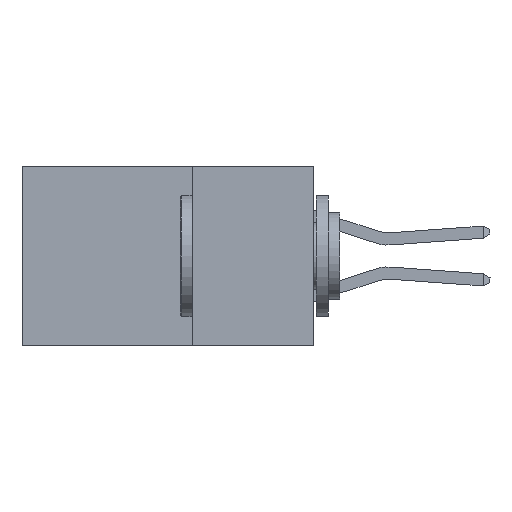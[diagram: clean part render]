
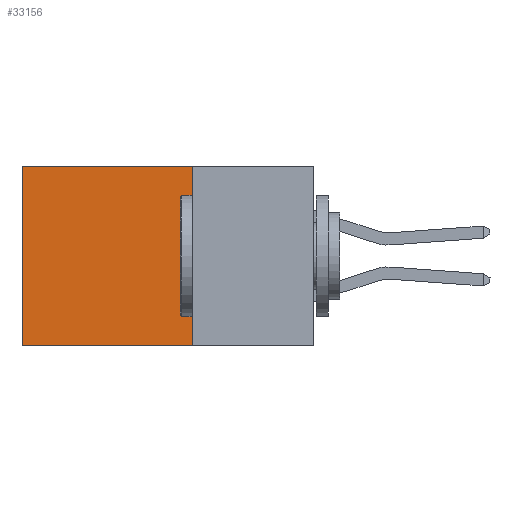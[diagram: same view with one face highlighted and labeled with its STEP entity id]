
A CAD part, left-side view. The second image highlights one B-rep face of the part: STEP entity #33156.
In plain terms, the highlighted planar face has unit normal (-1, 0, 0).
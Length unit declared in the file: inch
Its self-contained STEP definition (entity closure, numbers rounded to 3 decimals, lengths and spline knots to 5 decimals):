
#2 = LINE ( 'NONE', #2677, #33622 ) ;
#867 = CARTESIAN_POINT ( 'NONE',  ( 0.2875, 0.6, -0.37 ) ) ;
#2677 = CARTESIAN_POINT ( 'NONE',  ( 0.2875, 0.25, 0. ) ) ;
#4346 = CARTESIAN_POINT ( 'NONE',  ( 0.2875, 0.6, 0. ) ) ;
#4433 = FACE_OUTER_BOUND ( 'NONE', #28757, .T. ) ;
#5062 = VERTEX_POINT ( 'NONE', #21839 ) ;
#6774 = VERTEX_POINT ( 'NONE', #867 ) ;
#6911 = PLANE ( 'NONE',  #13733 ) ;
#7491 = CARTESIAN_POINT ( 'NONE',  ( 0.2875, 0.25, 0. ) ) ;
#7941 = EDGE_CURVE ( 'NONE', #5062, #6774, #16552, .T. ) ;
#8638 = VERTEX_POINT ( 'NONE', #34387 ) ;
#11840 = VECTOR ( 'NONE', #37527, 39.37008 ) ;
#12839 = CARTESIAN_POINT ( 'NONE',  ( 0.2875, 0.25, 0. ) ) ;
#12876 = LINE ( 'NONE', #27738, #34406 ) ;
#13670 = VERTEX_POINT ( 'NONE', #12839 ) ;
#13733 = AXIS2_PLACEMENT_3D ( 'NONE', #7491, #30981, #37150 ) ;
#14967 = ORIENTED_EDGE ( 'NONE', *, *, #7941, .T. ) ;
#16552 = LINE ( 'NONE', #4346, #11840 ) ;
#18169 = DIRECTION ( 'NONE',  ( 0., 0., -1. ) ) ;
#18315 = CARTESIAN_POINT ( 'NONE',  ( 0.2875, 0.25, 0. ) ) ;
#20875 = LINE ( 'NONE', #18315, #22999 ) ;
#21839 = CARTESIAN_POINT ( 'NONE',  ( 0.2875, 0.6, 0. ) ) ;
#22999 = VECTOR ( 'NONE', #18169, 39.37008 ) ;
#23665 = ORIENTED_EDGE ( 'NONE', *, *, #42968, .F. ) ;
#24610 = ORIENTED_EDGE ( 'NONE', *, *, #30571, .F. ) ;
#27738 = CARTESIAN_POINT ( 'NONE',  ( 0.2875, 0.25, -0.37 ) ) ;
#28757 = EDGE_LOOP ( 'NONE', ( #14967, #23665, #24610, #33577 ) ) ;
#30571 = EDGE_CURVE ( 'NONE', #13670, #8638, #20875, .T. ) ;
#30981 = DIRECTION ( 'NONE',  ( 1., 0., 0. ) ) ;
#33156 = ADVANCED_FACE ( 'NONE', ( #4433 ), #6911, .F. ) ;
#33577 = ORIENTED_EDGE ( 'NONE', *, *, #34767, .T. ) ;
#33622 = VECTOR ( 'NONE', #43020, 39.37008 ) ;
#34387 = CARTESIAN_POINT ( 'NONE',  ( 0.2875, 0.25, -0.37 ) ) ;
#34406 = VECTOR ( 'NONE', #35259, 39.37008 ) ;
#34767 = EDGE_CURVE ( 'NONE', #13670, #5062, #2, .T. ) ;
#35259 = DIRECTION ( 'NONE',  ( 0., 1., 0. ) ) ;
#37150 = DIRECTION ( 'NONE',  ( 0., 0., -1. ) ) ;
#37527 = DIRECTION ( 'NONE',  ( 0., 0., -1. ) ) ;
#42968 = EDGE_CURVE ( 'NONE', #8638, #6774, #12876, .T. ) ;
#43020 = DIRECTION ( 'NONE',  ( 0., 1., 0. ) ) ;
